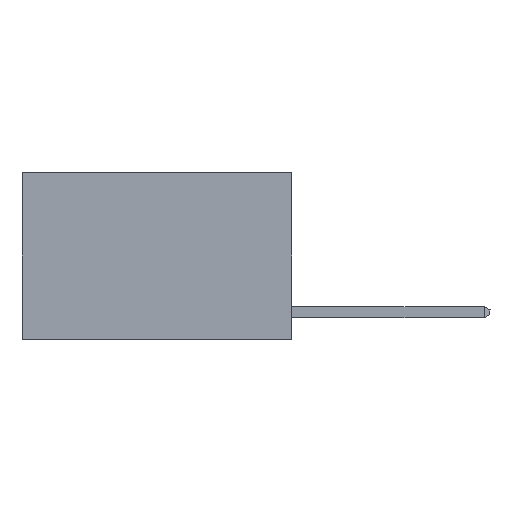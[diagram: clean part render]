
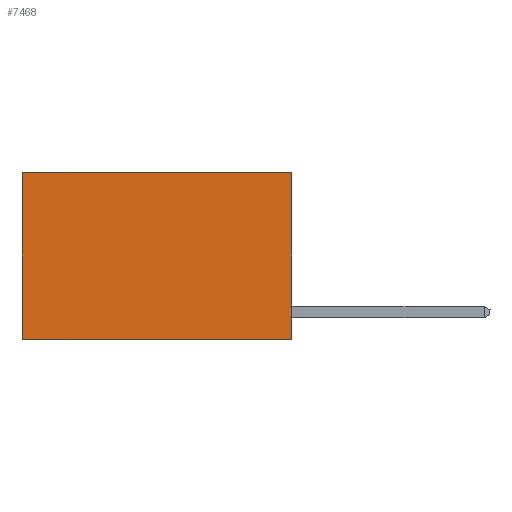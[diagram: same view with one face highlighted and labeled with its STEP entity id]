
A CAD part, left-side view. The second image highlights one B-rep face of the part: STEP entity #7468.
In plain terms, the highlighted planar face has unit normal (-1, 0, 0).
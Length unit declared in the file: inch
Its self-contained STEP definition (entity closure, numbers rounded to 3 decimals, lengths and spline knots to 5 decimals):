
#909 = PLANE ( 'NONE',  #13079 ) ;
#1435 = CARTESIAN_POINT ( 'NONE',  ( 0.2625, 0.6, -0.37 ) ) ;
#1875 = VERTEX_POINT ( 'NONE', #1435 ) ;
#3495 = VERTEX_POINT ( 'NONE', #9041 ) ;
#3638 = EDGE_CURVE ( 'NONE', #17229, #1875, #17879, .T. ) ;
#3714 = ORIENTED_EDGE ( 'NONE', *, *, #3638, .T. ) ;
#4134 = CARTESIAN_POINT ( 'NONE',  ( 0.2625, 0., 0. ) ) ;
#5855 = FACE_OUTER_BOUND ( 'NONE', #6531, .T. ) ;
#6251 = DIRECTION ( 'NONE',  ( 0., 0., -1. ) ) ;
#6531 = EDGE_LOOP ( 'NONE', ( #3714, #12002, #9907, #14405 ) ) ;
#6728 = CARTESIAN_POINT ( 'NONE',  ( 0.2625, 0., 0. ) ) ;
#7468 = ADVANCED_FACE ( 'NONE', ( #5855 ), #909, .F. ) ;
#7954 = VERTEX_POINT ( 'NONE', #8243 ) ;
#8243 = CARTESIAN_POINT ( 'NONE',  ( 0.2625, 0., 0. ) ) ;
#9041 = CARTESIAN_POINT ( 'NONE',  ( 0.2625, 0., -0.37 ) ) ;
#9529 = LINE ( 'NONE', #4134, #18965 ) ;
#9907 = ORIENTED_EDGE ( 'NONE', *, *, #18936, .F. ) ;
#10175 = EDGE_CURVE ( 'NONE', #3495, #1875, #18090, .T. ) ;
#10190 = DIRECTION ( 'NONE',  ( 1., 0., 0. ) ) ;
#10523 = DIRECTION ( 'NONE',  ( 0., 1., 0. ) ) ;
#11905 = EDGE_CURVE ( 'NONE', #7954, #17229, #15114, .T. ) ;
#12002 = ORIENTED_EDGE ( 'NONE', *, *, #10175, .F. ) ;
#13079 = AXIS2_PLACEMENT_3D ( 'NONE', #19019, #10190, #22598 ) ;
#14098 = CARTESIAN_POINT ( 'NONE',  ( 0.2625, 0., -0.37 ) ) ;
#14405 = ORIENTED_EDGE ( 'NONE', *, *, #11905, .T. ) ;
#14677 = CARTESIAN_POINT ( 'NONE',  ( 0.2625, 0.6, 0. ) ) ;
#14948 = DIRECTION ( 'NONE',  ( 0., 0., -1. ) ) ;
#15114 = LINE ( 'NONE', #6728, #22316 ) ;
#17229 = VERTEX_POINT ( 'NONE', #14677 ) ;
#17516 = VECTOR ( 'NONE', #10523, 39.37008 ) ;
#17879 = LINE ( 'NONE', #18467, #22030 ) ;
#18090 = LINE ( 'NONE', #14098, #17516 ) ;
#18467 = CARTESIAN_POINT ( 'NONE',  ( 0.2625, 0.6, 0. ) ) ;
#18936 = EDGE_CURVE ( 'NONE', #7954, #3495, #9529, .T. ) ;
#18965 = VECTOR ( 'NONE', #14948, 39.37008 ) ;
#19019 = CARTESIAN_POINT ( 'NONE',  ( 0.2625, 0., 0. ) ) ;
#21012 = DIRECTION ( 'NONE',  ( 0., 1., 0. ) ) ;
#22030 = VECTOR ( 'NONE', #6251, 39.37008 ) ;
#22316 = VECTOR ( 'NONE', #21012, 39.37008 ) ;
#22598 = DIRECTION ( 'NONE',  ( 0., 0., -1. ) ) ;
